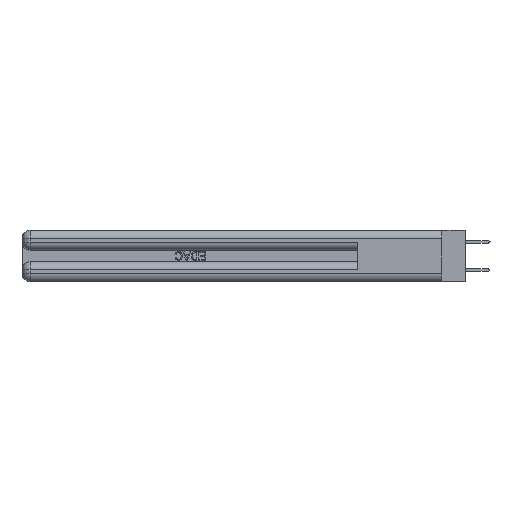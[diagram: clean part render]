
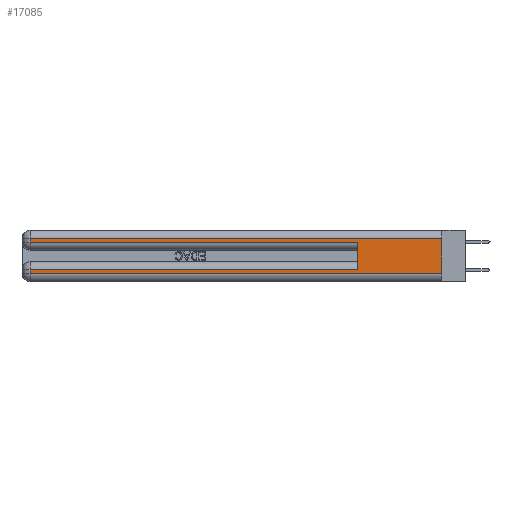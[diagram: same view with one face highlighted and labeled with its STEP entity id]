
A CAD part, left-side view. The second image highlights one B-rep face of the part: STEP entity #17085.
In plain terms, the highlighted planar face has unit normal (-1, 0, 0).
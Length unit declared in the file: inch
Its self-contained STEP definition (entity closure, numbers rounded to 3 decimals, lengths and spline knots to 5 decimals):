
#650 = CARTESIAN_POINT ( 'NONE',  ( 0., 2.94, 0.285 ) ) ;
#2197 = LINE ( 'NONE', #17176, #16012 ) ;
#2562 = VECTOR ( 'NONE', #9163, 39.37008 ) ;
#3052 = EDGE_CURVE ( 'NONE', #32906, #19036, #4809, .T. ) ;
#4098 = EDGE_CURVE ( 'NONE', #8633, #32906, #30064, .T. ) ;
#4149 = LINE ( 'NONE', #30525, #2562 ) ;
#4165 = CARTESIAN_POINT ( 'NONE',  ( 0., 0.6, 0.145 ) ) ;
#4593 = CARTESIAN_POINT ( 'NONE',  ( 0., 0., 0.37 ) ) ;
#4809 = LINE ( 'NONE', #25452, #40138 ) ;
#5468 = CARTESIAN_POINT ( 'NONE',  ( 0., 2.94, 0.085 ) ) ;
#5525 = CARTESIAN_POINT ( 'NONE',  ( 0., 0.6, 0.085 ) ) ;
#6642 = ORIENTED_EDGE ( 'NONE', *, *, #36210, .T. ) ;
#6692 = LINE ( 'NONE', #39910, #43073 ) ;
#6975 = ORIENTED_EDGE ( 'NONE', *, *, #3052, .T. ) ;
#7451 = EDGE_CURVE ( 'NONE', #32590, #35949, #6692, .T. ) ;
#8118 = DIRECTION ( 'NONE',  ( 0., 0., -1. ) ) ;
#8633 = VERTEX_POINT ( 'NONE', #19394 ) ;
#8769 = ORIENTED_EDGE ( 'NONE', *, *, #34187, .F. ) ;
#9163 = DIRECTION ( 'NONE',  ( 0., 0., -1. ) ) ;
#10303 = ORIENTED_EDGE ( 'NONE', *, *, #4098, .T. ) ;
#10351 = EDGE_CURVE ( 'NONE', #35949, #27954, #24338, .T. ) ;
#10385 = CARTESIAN_POINT ( 'NONE',  ( 0., 2.94, 0.37 ) ) ;
#11458 = DIRECTION ( 'NONE',  ( 0., -1., 0. ) ) ;
#11481 = DIRECTION ( 'NONE',  ( 0., -1., 0. ) ) ;
#11840 = PLANE ( 'NONE',  #38667 ) ;
#15522 = CARTESIAN_POINT ( 'NONE',  ( 0., 2.94, 0.37 ) ) ;
#16012 = VECTOR ( 'NONE', #17736, 39.37008 ) ;
#16061 = EDGE_LOOP ( 'NONE', ( #8769, #6642, #10303, #6975, #21045, #22846, #33168, #36900 ) ) ;
#17085 = ADVANCED_FACE ( 'NONE', ( #37785 ), #11840, .F. ) ;
#17176 = CARTESIAN_POINT ( 'NONE',  ( 0., 0., 0.31 ) ) ;
#17304 = DIRECTION ( 'NONE',  ( 0., 0., 1. ) ) ;
#17472 = DIRECTION ( 'NONE',  ( 0., 0., -1. ) ) ;
#17736 = DIRECTION ( 'NONE',  ( 0., 1., 0. ) ) ;
#18396 = CARTESIAN_POINT ( 'NONE',  ( 0., 0., 0.06 ) ) ;
#19036 = VERTEX_POINT ( 'NONE', #29673 ) ;
#19394 = CARTESIAN_POINT ( 'NONE',  ( 0., 2.94, 0.31 ) ) ;
#20698 = VECTOR ( 'NONE', #17472, 39.37008 ) ;
#21045 = ORIENTED_EDGE ( 'NONE', *, *, #26921, .F. ) ;
#22293 = DIRECTION ( 'NONE',  ( 0., 1., 0. ) ) ;
#22846 = ORIENTED_EDGE ( 'NONE', *, *, #7451, .T. ) ;
#23376 = LINE ( 'NONE', #4165, #37189 ) ;
#23425 = VERTEX_POINT ( 'NONE', #26238 ) ;
#24338 = LINE ( 'NONE', #15522, #38191 ) ;
#24435 = CARTESIAN_POINT ( 'NONE',  ( 0., 0., 0.31 ) ) ;
#25125 = VECTOR ( 'NONE', #11481, 39.37008 ) ;
#25147 = EDGE_CURVE ( 'NONE', #27954, #23425, #42807, .T. ) ;
#25452 = CARTESIAN_POINT ( 'NONE',  ( 0., 0., 0.285 ) ) ;
#26238 = CARTESIAN_POINT ( 'NONE',  ( 0., 0., 0.06 ) ) ;
#26505 = CARTESIAN_POINT ( 'NONE',  ( 0., 2.94, 0.06 ) ) ;
#26921 = EDGE_CURVE ( 'NONE', #32590, #19036, #23376, .T. ) ;
#27954 = VERTEX_POINT ( 'NONE', #26505 ) ;
#29160 = DIRECTION ( 'NONE',  ( 0., 0., -1. ) ) ;
#29219 = DIRECTION ( 'NONE',  ( 1., 0., 0. ) ) ;
#29673 = CARTESIAN_POINT ( 'NONE',  ( 0., 0.6, 0.285 ) ) ;
#30064 = LINE ( 'NONE', #10385, #20698 ) ;
#30525 = CARTESIAN_POINT ( 'NONE',  ( 0., 0., 0.37 ) ) ;
#32590 = VERTEX_POINT ( 'NONE', #5525 ) ;
#32906 = VERTEX_POINT ( 'NONE', #650 ) ;
#33168 = ORIENTED_EDGE ( 'NONE', *, *, #10351, .T. ) ;
#33738 = VERTEX_POINT ( 'NONE', #24435 ) ;
#34187 = EDGE_CURVE ( 'NONE', #33738, #23425, #4149, .T. ) ;
#35949 = VERTEX_POINT ( 'NONE', #5468 ) ;
#36210 = EDGE_CURVE ( 'NONE', #33738, #8633, #2197, .T. ) ;
#36900 = ORIENTED_EDGE ( 'NONE', *, *, #25147, .T. ) ;
#37189 = VECTOR ( 'NONE', #17304, 39.37008 ) ;
#37785 = FACE_OUTER_BOUND ( 'NONE', #16061, .T. ) ;
#38191 = VECTOR ( 'NONE', #29160, 39.37008 ) ;
#38667 = AXIS2_PLACEMENT_3D ( 'NONE', #4593, #29219, #8118 ) ;
#39910 = CARTESIAN_POINT ( 'NONE',  ( 0., 0., 0.085 ) ) ;
#40138 = VECTOR ( 'NONE', #11458, 39.37008 ) ;
#42807 = LINE ( 'NONE', #18396, #25125 ) ;
#43073 = VECTOR ( 'NONE', #22293, 39.37008 ) ;
